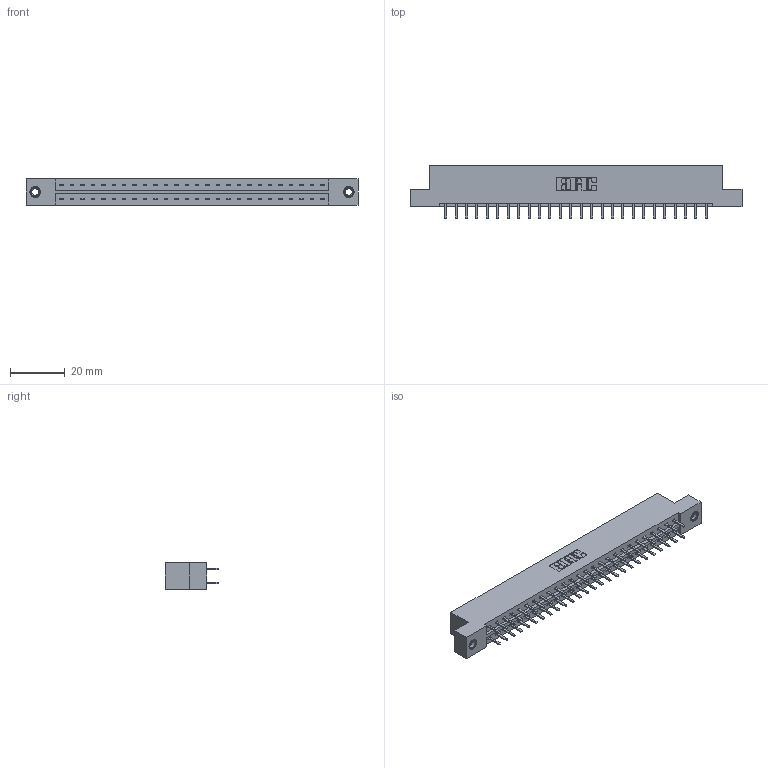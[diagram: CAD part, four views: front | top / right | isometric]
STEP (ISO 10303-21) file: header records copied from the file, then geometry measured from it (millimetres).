
FILE_DESCRIPTION (( 'STEP AP203' ), '1' );
FILE_NAME ('379-052-520-207.STEP', '2020-02-26T17:29:34', ( '' ), ( '' ), 'SwSTEP 2.0', 'SolidWorks 2016', '' );
FILE_SCHEMA (( 'CONFIG_CONTROL_DESIGN' ));
Length unit declared in the file: inch
Products named in the file (4): 379-052-520-207; 345-250-001_345-250-005-103; 379 Part_Flush - .156 Dia - TI; 345-292-001_345-293-120
Assembly tree (55 placements, depth 2):
  379-052-520-207
    379 Part_Flush - .156 Dia - TI
    345-292-001_345-293-120  x52
    345-250-001_345-250-005-103  x2
Bounding box: 121.28 x 19.68 x 9.53 mm (x, y, z)
Volume: 12685.8 mm3; surface area: 14072.3 mm2
Topology: 55 solids, 55 shells, 3086 faces, 8923 edges, 5802 vertices
Faces by surface type: plane 2078, cylinder 992, cone 12, torus 4
Entity records: 20096 total; most frequent: CARTESIAN_POINT 3345, ORIENTED_EDGE 3262, DIRECTION 2905, EDGE_CURVE 1631, LINE 1479, VECTOR 1479, VERTEX_POINT 1080, AXIS2_PLACEMENT_3D 713
